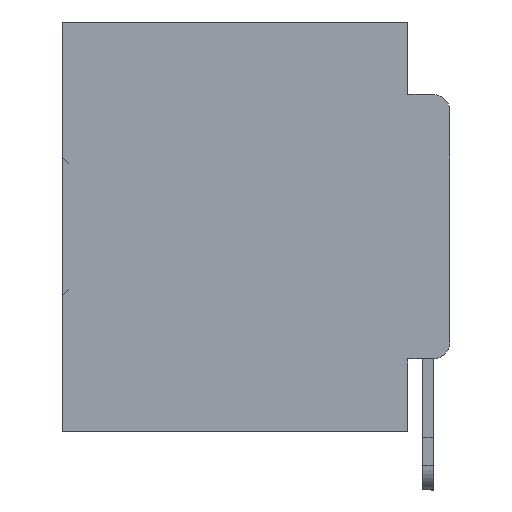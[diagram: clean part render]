
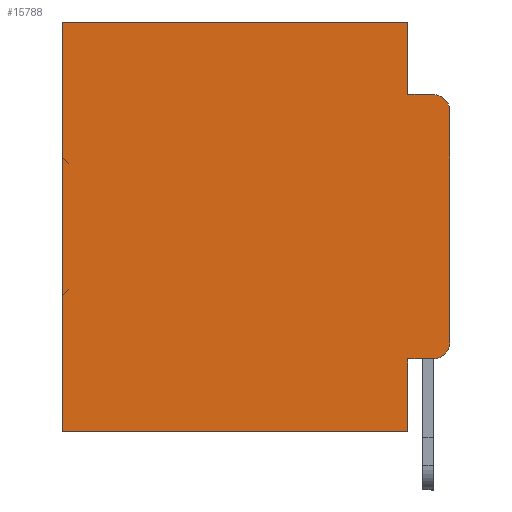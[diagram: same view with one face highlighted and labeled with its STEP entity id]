
A CAD part, left-side view. The second image highlights one B-rep face of the part: STEP entity #15788.
In plain terms, the highlighted planar face has unit normal (-1, 0, 0).
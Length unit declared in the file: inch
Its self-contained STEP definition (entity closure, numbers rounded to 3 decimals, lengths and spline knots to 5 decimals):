
#708 = ORIENTED_EDGE ( 'NONE', *, *, #3754, .T. ) ;
#1570 = LINE ( 'NONE', #9938, #17944 ) ;
#1892 = CARTESIAN_POINT ( 'NONE',  ( 0.298, 0., -0.1085 ) ) ;
#2052 = CARTESIAN_POINT ( 'NONE',  ( 0.298, 0.051, -0.4115 ) ) ;
#2089 = LINE ( 'NONE', #2450, #13149 ) ;
#2450 = CARTESIAN_POINT ( 'NONE',  ( 0.298, 0.473, 0. ) ) ;
#2947 = DIRECTION ( 'NONE',  ( 0., 1., 0. ) ) ;
#3135 = LINE ( 'NONE', #28398, #33633 ) ;
#3426 = DIRECTION ( 'NONE',  ( 0., 0., -1. ) ) ;
#3754 = EDGE_CURVE ( 'NONE', #11282, #26905, #33748, .T. ) ;
#4157 = CARTESIAN_POINT ( 'NONE',  ( 0.298, 0., -0.3915 ) ) ;
#4533 = ORIENTED_EDGE ( 'NONE', *, *, #23704, .T. ) ;
#4651 = EDGE_LOOP ( 'NONE', ( #26555, #4533, #27516, #34963, #22214, #5107, #6424, #8776, #708, #19294 ) ) ;
#5107 = ORIENTED_EDGE ( 'NONE', *, *, #24121, .T. ) ;
#5573 = CARTESIAN_POINT ( 'NONE',  ( 0.298, 0.473, -0.5 ) ) ;
#5920 = VERTEX_POINT ( 'NONE', #9236 ) ;
#6217 = CARTESIAN_POINT ( 'NONE',  ( 0.298, 0.051, 0. ) ) ;
#6335 = EDGE_CURVE ( 'NONE', #22806, #13447, #25554, .T. ) ;
#6424 = ORIENTED_EDGE ( 'NONE', *, *, #36300, .F. ) ;
#7384 = DIRECTION ( 'NONE',  ( -1., 0., 0. ) ) ;
#8257 = LINE ( 'NONE', #27761, #11568 ) ;
#8509 = DIRECTION ( 'NONE',  ( 0., 0., -1. ) ) ;
#8613 = DIRECTION ( 'NONE',  ( 0., 1., 0. ) ) ;
#8776 = ORIENTED_EDGE ( 'NONE', *, *, #15097, .F. ) ;
#8807 = EDGE_CURVE ( 'NONE', #24135, #18658, #10768, .T. ) ;
#8843 = AXIS2_PLACEMENT_3D ( 'NONE', #10933, #30803, #8509 ) ;
#9236 = CARTESIAN_POINT ( 'NONE',  ( 0.298, 0.051, -0.5 ) ) ;
#9938 = CARTESIAN_POINT ( 'NONE',  ( 0.298, 0.051, -0.0885 ) ) ;
#10204 = VERTEX_POINT ( 'NONE', #31353 ) ;
#10216 = DIRECTION ( 'NONE',  ( 0., 0., -1. ) ) ;
#10278 = VECTOR ( 'NONE', #10216, 39.37008 ) ;
#10768 = LINE ( 'NONE', #27661, #10278 ) ;
#10852 = VECTOR ( 'NONE', #36349, 39.37008 ) ;
#10933 = CARTESIAN_POINT ( 'NONE',  ( 0.298, 0., 0. ) ) ;
#11282 = VERTEX_POINT ( 'NONE', #2052 ) ;
#11568 = VECTOR ( 'NONE', #8613, 39.37008 ) ;
#11941 = CIRCLE ( 'NONE', #17861, 0.02 ) ;
#11983 = DIRECTION ( 'NONE',  ( 0., 0., -1. ) ) ;
#13149 = VECTOR ( 'NONE', #16399, 39.37008 ) ;
#13447 = VERTEX_POINT ( 'NONE', #4157 ) ;
#15097 = EDGE_CURVE ( 'NONE', #11282, #5920, #35281, .T. ) ;
#15788 = ADVANCED_FACE ( 'NONE', ( #28372 ), #30979, .F. ) ;
#15850 = CARTESIAN_POINT ( 'NONE',  ( 0.298, 0.02, -0.4115 ) ) ;
#16399 = DIRECTION ( 'NONE',  ( 0., 0., -1. ) ) ;
#16458 = AXIS2_PLACEMENT_3D ( 'NONE', #24665, #7384, #18900 ) ;
#17861 = AXIS2_PLACEMENT_3D ( 'NONE', #29211, #34933, #18251 ) ;
#17863 = EDGE_CURVE ( 'NONE', #26905, #13447, #11941, .T. ) ;
#17944 = VECTOR ( 'NONE', #35161, 39.37008 ) ;
#18251 = DIRECTION ( 'NONE',  ( 0., 0., -1. ) ) ;
#18658 = VERTEX_POINT ( 'NONE', #28379 ) ;
#18900 = DIRECTION ( 'NONE',  ( 0., 0., -1. ) ) ;
#19294 = ORIENTED_EDGE ( 'NONE', *, *, #17863, .T. ) ;
#22214 = ORIENTED_EDGE ( 'NONE', *, *, #29027, .T. ) ;
#22806 = VERTEX_POINT ( 'NONE', #1892 ) ;
#23704 = EDGE_CURVE ( 'NONE', #22806, #24691, #32428, .T. ) ;
#24121 = EDGE_CURVE ( 'NONE', #10204, #36269, #2089, .T. ) ;
#24135 = VERTEX_POINT ( 'NONE', #35856 ) ;
#24665 = CARTESIAN_POINT ( 'NONE',  ( 0.298, 0.02, -0.1085 ) ) ;
#24691 = VERTEX_POINT ( 'NONE', #25949 ) ;
#25554 = LINE ( 'NONE', #28336, #28759 ) ;
#25949 = CARTESIAN_POINT ( 'NONE',  ( 0.298, 0.02, -0.0885 ) ) ;
#26469 = EDGE_CURVE ( 'NONE', #18658, #24691, #1570, .T. ) ;
#26555 = ORIENTED_EDGE ( 'NONE', *, *, #6335, .F. ) ;
#26905 = VERTEX_POINT ( 'NONE', #15850 ) ;
#27516 = ORIENTED_EDGE ( 'NONE', *, *, #26469, .F. ) ;
#27661 = CARTESIAN_POINT ( 'NONE',  ( 0.298, 0.051, 0. ) ) ;
#27761 = CARTESIAN_POINT ( 'NONE',  ( 0.298, 0., 0. ) ) ;
#28336 = CARTESIAN_POINT ( 'NONE',  ( 0.298, 0., 0. ) ) ;
#28372 = FACE_OUTER_BOUND ( 'NONE', #4651, .T. ) ;
#28379 = CARTESIAN_POINT ( 'NONE',  ( 0.298, 0.051, -0.0885 ) ) ;
#28398 = CARTESIAN_POINT ( 'NONE',  ( 0.298, 0., -0.5 ) ) ;
#28759 = VECTOR ( 'NONE', #11983, 39.37008 ) ;
#29027 = EDGE_CURVE ( 'NONE', #24135, #10204, #8257, .T. ) ;
#29211 = CARTESIAN_POINT ( 'NONE',  ( 0.298, 0.02, -0.3915 ) ) ;
#30803 = DIRECTION ( 'NONE',  ( 1., 0., 0. ) ) ;
#30808 = CARTESIAN_POINT ( 'NONE',  ( 0.298, 0.051, -0.4115 ) ) ;
#30979 = PLANE ( 'NONE',  #8843 ) ;
#31353 = CARTESIAN_POINT ( 'NONE',  ( 0.298, 0.473, 0. ) ) ;
#32428 = CIRCLE ( 'NONE', #16458, 0.02 ) ;
#33633 = VECTOR ( 'NONE', #2947, 39.37008 ) ;
#33748 = LINE ( 'NONE', #30808, #10852 ) ;
#34877 = VECTOR ( 'NONE', #3426, 39.37008 ) ;
#34933 = DIRECTION ( 'NONE',  ( -1., 0., 0. ) ) ;
#34963 = ORIENTED_EDGE ( 'NONE', *, *, #8807, .F. ) ;
#35161 = DIRECTION ( 'NONE',  ( 0., -1., 0. ) ) ;
#35281 = LINE ( 'NONE', #6217, #34877 ) ;
#35856 = CARTESIAN_POINT ( 'NONE',  ( 0.298, 0.051, 0. ) ) ;
#36269 = VERTEX_POINT ( 'NONE', #5573 ) ;
#36300 = EDGE_CURVE ( 'NONE', #5920, #36269, #3135, .T. ) ;
#36349 = DIRECTION ( 'NONE',  ( 0., -1., 0. ) ) ;
